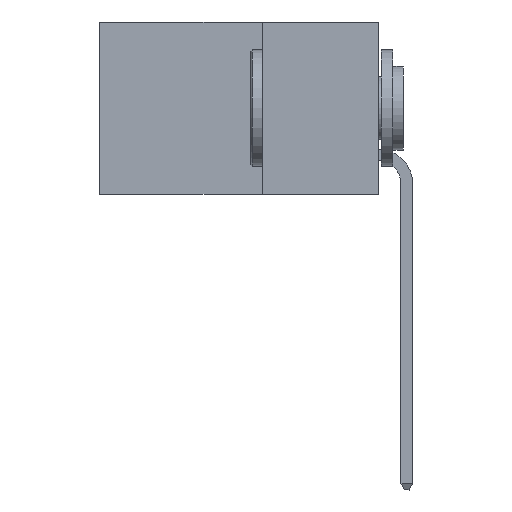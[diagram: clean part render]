
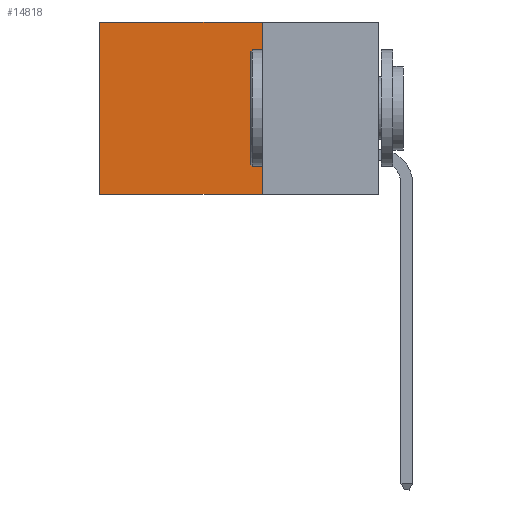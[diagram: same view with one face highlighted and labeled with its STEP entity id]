
A CAD part, left-side view. The second image highlights one B-rep face of the part: STEP entity #14818.
In plain terms, the highlighted planar face has unit normal (-1, 0, 0).
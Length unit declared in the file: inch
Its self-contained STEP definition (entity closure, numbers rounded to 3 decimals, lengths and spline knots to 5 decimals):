
#135 = CARTESIAN_POINT ( 'NONE',  ( 0.2615, 0.6, 0. ) ) ;
#218 = EDGE_CURVE ( 'NONE', #17352, #2645, #11233, .T. ) ;
#1283 = DIRECTION ( 'NONE',  ( 0., 0., -1. ) ) ;
#2645 = VERTEX_POINT ( 'NONE', #13407 ) ;
#3311 = EDGE_LOOP ( 'NONE', ( #5822, #6955, #12386, #18384 ) ) ;
#3711 = CARTESIAN_POINT ( 'NONE',  ( 0.2615, 0.25, 0. ) ) ;
#4065 = VERTEX_POINT ( 'NONE', #9209 ) ;
#5822 = ORIENTED_EDGE ( 'NONE', *, *, #16717, .T. ) ;
#6344 = VERTEX_POINT ( 'NONE', #135 ) ;
#6376 = CARTESIAN_POINT ( 'NONE',  ( 0.2615, 0.25, 0. ) ) ;
#6754 = LINE ( 'NONE', #12503, #16170 ) ;
#6871 = EDGE_CURVE ( 'NONE', #17352, #6344, #7810, .T. ) ;
#6896 = AXIS2_PLACEMENT_3D ( 'NONE', #8329, #9457, #14058 ) ;
#6955 = ORIENTED_EDGE ( 'NONE', *, *, #9487, .F. ) ;
#7810 = LINE ( 'NONE', #3711, #17157 ) ;
#8329 = CARTESIAN_POINT ( 'NONE',  ( 0.2615, 0.25, -0.37 ) ) ;
#9209 = CARTESIAN_POINT ( 'NONE',  ( 0.2615, 0.6, -0.37 ) ) ;
#9414 = VECTOR ( 'NONE', #1283, 39.37008 ) ;
#9457 = DIRECTION ( 'NONE',  ( 1., 0., 0. ) ) ;
#9487 = EDGE_CURVE ( 'NONE', #2645, #4065, #6754, .T. ) ;
#9588 = DIRECTION ( 'NONE',  ( 0., 1., 0. ) ) ;
#9634 = CARTESIAN_POINT ( 'NONE',  ( 0.2615, 0.25, -0.37 ) ) ;
#9741 = PLANE ( 'NONE',  #6896 ) ;
#10369 = DIRECTION ( 'NONE',  ( 0., 0., -1. ) ) ;
#11095 = DIRECTION ( 'NONE',  ( 0., 1., 0. ) ) ;
#11233 = LINE ( 'NONE', #9634, #9414 ) ;
#12386 = ORIENTED_EDGE ( 'NONE', *, *, #218, .F. ) ;
#12503 = CARTESIAN_POINT ( 'NONE',  ( 0.2615, 0.25, -0.37 ) ) ;
#13189 = LINE ( 'NONE', #16228, #13873 ) ;
#13407 = CARTESIAN_POINT ( 'NONE',  ( 0.2615, 0.25, -0.37 ) ) ;
#13873 = VECTOR ( 'NONE', #10369, 39.37008 ) ;
#14058 = DIRECTION ( 'NONE',  ( 0., 0., -1. ) ) ;
#14818 = ADVANCED_FACE ( 'NONE', ( #16927 ), #9741, .F. ) ;
#16170 = VECTOR ( 'NONE', #11095, 39.37008 ) ;
#16228 = CARTESIAN_POINT ( 'NONE',  ( 0.2615, 0.6, -0.37 ) ) ;
#16717 = EDGE_CURVE ( 'NONE', #6344, #4065, #13189, .T. ) ;
#16927 = FACE_OUTER_BOUND ( 'NONE', #3311, .T. ) ;
#17157 = VECTOR ( 'NONE', #9588, 39.37008 ) ;
#17352 = VERTEX_POINT ( 'NONE', #6376 ) ;
#18384 = ORIENTED_EDGE ( 'NONE', *, *, #6871, .T. ) ;
